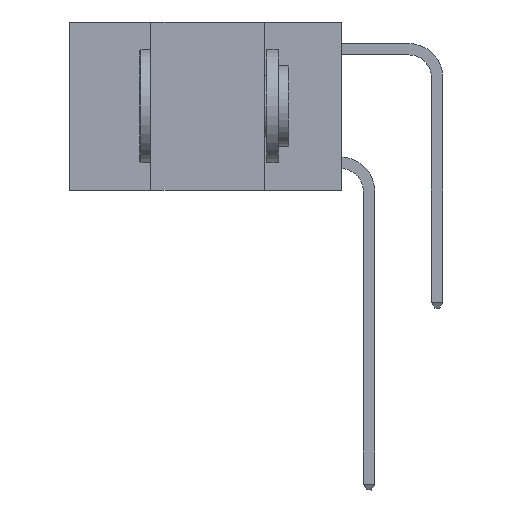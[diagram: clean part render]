
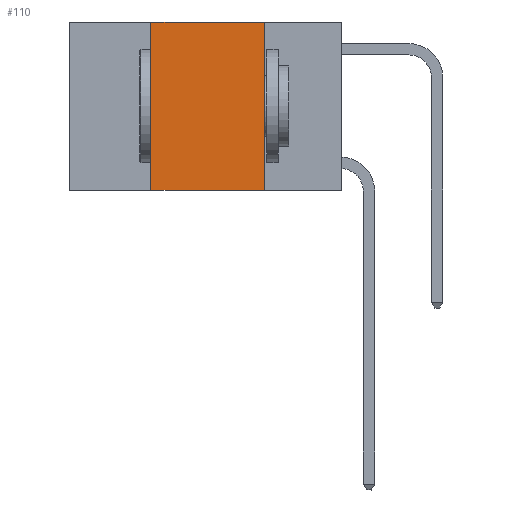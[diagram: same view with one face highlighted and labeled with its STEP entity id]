
A CAD part, left-side view. The second image highlights one B-rep face of the part: STEP entity #110.
In plain terms, the highlighted planar face has unit normal (-1, 0, 0).
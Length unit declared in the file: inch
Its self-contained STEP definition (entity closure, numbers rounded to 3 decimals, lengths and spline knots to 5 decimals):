
#110 = ADVANCED_FACE ( 'NONE', ( #16976 ), #12839, .F. ) ;
#173 = LINE ( 'NONE', #23133, #9613 ) ;
#624 = VECTOR ( 'NONE', #12935, 39.37008 ) ;
#938 = LINE ( 'NONE', #20688, #6795 ) ;
#1350 = CARTESIAN_POINT ( 'NONE',  ( 0., 0.42, 0. ) ) ;
#1783 = ORIENTED_EDGE ( 'NONE', *, *, #6589, .F. ) ;
#2844 = AXIS2_PLACEMENT_3D ( 'NONE', #3372, #5023, #8891 ) ;
#3372 = CARTESIAN_POINT ( 'NONE',  ( 0., 0.6, 0. ) ) ;
#3455 = CARTESIAN_POINT ( 'NONE',  ( 0., 0.42, -0.37 ) ) ;
#4821 = EDGE_LOOP ( 'NONE', ( #7171, #20220, #1783, #22863 ) ) ;
#5023 = DIRECTION ( 'NONE',  ( 1., 0., 0. ) ) ;
#5113 = CARTESIAN_POINT ( 'NONE',  ( 0., 0.17, 0. ) ) ;
#5712 = EDGE_CURVE ( 'NONE', #10617, #14821, #22573, .T. ) ;
#6077 = CARTESIAN_POINT ( 'NONE',  ( 0., 0.17, -0.37 ) ) ;
#6495 = DIRECTION ( 'NONE',  ( 0., -1., 0. ) ) ;
#6589 = EDGE_CURVE ( 'NONE', #14153, #10687, #938, .T. ) ;
#6795 = VECTOR ( 'NONE', #6954, 39.37008 ) ;
#6954 = DIRECTION ( 'NONE',  ( 0., 0., 1. ) ) ;
#7171 = ORIENTED_EDGE ( 'NONE', *, *, #5712, .F. ) ;
#8891 = DIRECTION ( 'NONE',  ( 0., 0., -1. ) ) ;
#9056 = EDGE_CURVE ( 'NONE', #10687, #10617, #18055, .T. ) ;
#9613 = VECTOR ( 'NONE', #13858, 39.37008 ) ;
#10617 = VERTEX_POINT ( 'NONE', #22397 ) ;
#10687 = VERTEX_POINT ( 'NONE', #1350 ) ;
#12543 = VECTOR ( 'NONE', #6495, 39.37008 ) ;
#12839 = PLANE ( 'NONE',  #2844 ) ;
#12935 = DIRECTION ( 'NONE',  ( 0., 0., -1. ) ) ;
#13858 = DIRECTION ( 'NONE',  ( 0., -1., 0. ) ) ;
#14153 = VERTEX_POINT ( 'NONE', #3455 ) ;
#14154 = CARTESIAN_POINT ( 'NONE',  ( 0., 0.6, 0. ) ) ;
#14821 = VERTEX_POINT ( 'NONE', #6077 ) ;
#16976 = FACE_OUTER_BOUND ( 'NONE', #4821, .T. ) ;
#18055 = LINE ( 'NONE', #14154, #12543 ) ;
#19883 = EDGE_CURVE ( 'NONE', #14153, #14821, #173, .T. ) ;
#20220 = ORIENTED_EDGE ( 'NONE', *, *, #9056, .F. ) ;
#20688 = CARTESIAN_POINT ( 'NONE',  ( 0., 0.42, 0. ) ) ;
#22397 = CARTESIAN_POINT ( 'NONE',  ( 0., 0.17, 0. ) ) ;
#22573 = LINE ( 'NONE', #5113, #624 ) ;
#22863 = ORIENTED_EDGE ( 'NONE', *, *, #19883, .T. ) ;
#23133 = CARTESIAN_POINT ( 'NONE',  ( 0., 0.6, -0.37 ) ) ;
